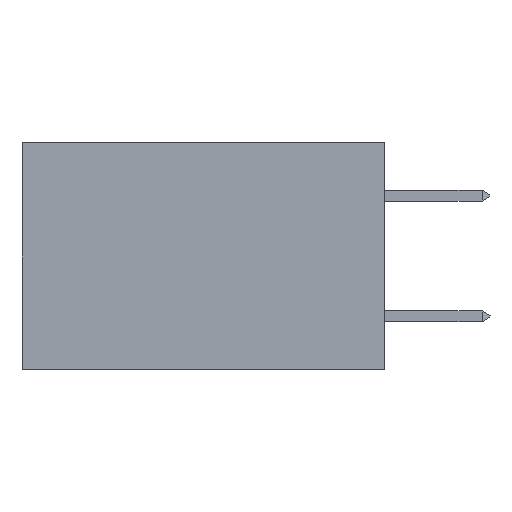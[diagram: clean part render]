
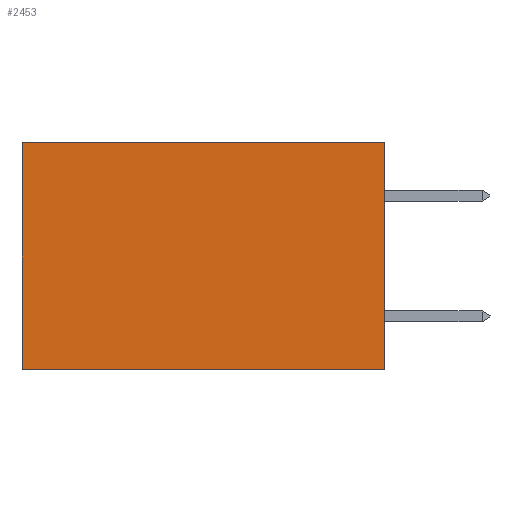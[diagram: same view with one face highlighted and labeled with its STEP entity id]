
A CAD part, left-side view. The second image highlights one B-rep face of the part: STEP entity #2453.
In plain terms, the highlighted planar face has unit normal (-1, 0, 0).
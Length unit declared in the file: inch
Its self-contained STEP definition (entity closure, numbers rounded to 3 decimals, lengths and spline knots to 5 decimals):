
#71 = ORIENTED_EDGE ( 'NONE', *, *, #3107, .F. ) ;
#265 = DIRECTION ( 'NONE',  ( 0., 1., 0. ) ) ;
#905 = EDGE_CURVE ( 'NONE', #14043, #2326, #12294, .T. ) ;
#1092 = LINE ( 'NONE', #8361, #4679 ) ;
#1365 = PLANE ( 'NONE',  #9930 ) ;
#1486 = LINE ( 'NONE', #8673, #6576 ) ;
#2326 = VERTEX_POINT ( 'NONE', #4933 ) ;
#2453 = ADVANCED_FACE ( 'NONE', ( #7169 ), #1365, .F. ) ;
#2795 = VECTOR ( 'NONE', #7917, 39.37008 ) ;
#3107 = EDGE_CURVE ( 'NONE', #10402, #14043, #1486, .T. ) ;
#4679 = VECTOR ( 'NONE', #9721, 39.37008 ) ;
#4899 = EDGE_LOOP ( 'NONE', ( #6154, #13721, #71, #5670 ) ) ;
#4933 = CARTESIAN_POINT ( 'NONE',  ( 0.2875, 0.6, -0.375 ) ) ;
#5372 = CARTESIAN_POINT ( 'NONE',  ( 0.2875, 0., 0. ) ) ;
#5484 = CARTESIAN_POINT ( 'NONE',  ( 0.2875, 0., -0.375 ) ) ;
#5670 = ORIENTED_EDGE ( 'NONE', *, *, #7772, .T. ) ;
#6154 = ORIENTED_EDGE ( 'NONE', *, *, #7489, .T. ) ;
#6268 = DIRECTION ( 'NONE',  ( 0., 0., -1. ) ) ;
#6576 = VECTOR ( 'NONE', #11155, 39.37008 ) ;
#6702 = CARTESIAN_POINT ( 'NONE',  ( 0.2875, 0., 0. ) ) ;
#7169 = FACE_OUTER_BOUND ( 'NONE', #4899, .T. ) ;
#7489 = EDGE_CURVE ( 'NONE', #8330, #2326, #1092, .T. ) ;
#7772 = EDGE_CURVE ( 'NONE', #10402, #8330, #8665, .T. ) ;
#7917 = DIRECTION ( 'NONE',  ( 0., 1., 0. ) ) ;
#8330 = VERTEX_POINT ( 'NONE', #9774 ) ;
#8361 = CARTESIAN_POINT ( 'NONE',  ( 0.2875, 0.6, -0.375 ) ) ;
#8665 = LINE ( 'NONE', #6702, #2795 ) ;
#8673 = CARTESIAN_POINT ( 'NONE',  ( 0.2875, 0., -0.375 ) ) ;
#8801 = CARTESIAN_POINT ( 'NONE',  ( 0.2875, 0., -0.375 ) ) ;
#9721 = DIRECTION ( 'NONE',  ( 0., 0., -1. ) ) ;
#9774 = CARTESIAN_POINT ( 'NONE',  ( 0.2875, 0.6, 0. ) ) ;
#9849 = DIRECTION ( 'NONE',  ( 1., 0., 0. ) ) ;
#9930 = AXIS2_PLACEMENT_3D ( 'NONE', #8801, #9849, #6268 ) ;
#10402 = VERTEX_POINT ( 'NONE', #5372 ) ;
#10408 = VECTOR ( 'NONE', #265, 39.37008 ) ;
#11155 = DIRECTION ( 'NONE',  ( 0., 0., -1. ) ) ;
#12294 = LINE ( 'NONE', #14678, #10408 ) ;
#13721 = ORIENTED_EDGE ( 'NONE', *, *, #905, .F. ) ;
#14043 = VERTEX_POINT ( 'NONE', #5484 ) ;
#14678 = CARTESIAN_POINT ( 'NONE',  ( 0.2875, 0., -0.375 ) ) ;
